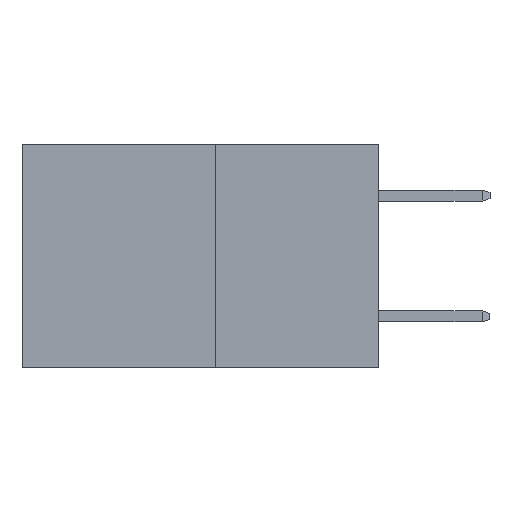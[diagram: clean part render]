
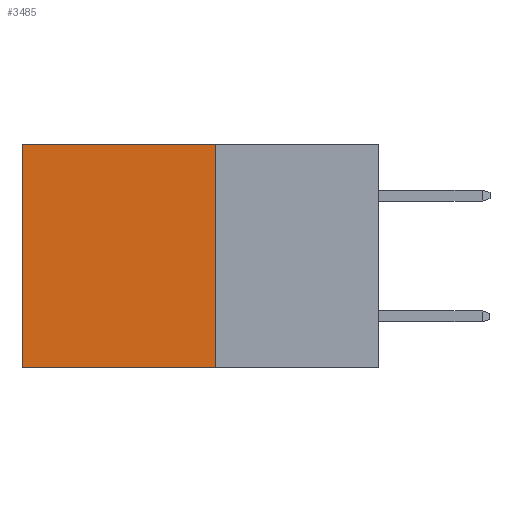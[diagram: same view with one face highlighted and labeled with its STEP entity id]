
A CAD part, left-side view. The second image highlights one B-rep face of the part: STEP entity #3485.
In plain terms, the highlighted planar face has unit normal (-1, 0, 0).
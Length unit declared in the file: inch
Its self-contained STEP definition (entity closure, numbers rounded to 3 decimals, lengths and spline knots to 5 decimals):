
#40 = DIRECTION ( 'NONE',  ( 1., 0., 0. ) ) ;
#182 = VECTOR ( 'NONE', #1301, 39.37008 ) ;
#316 = ORIENTED_EDGE ( 'NONE', *, *, #8505, .F. ) ;
#333 = VERTEX_POINT ( 'NONE', #3322 ) ;
#630 = EDGE_CURVE ( 'NONE', #333, #5329, #3388, .T. ) ;
#726 = DIRECTION ( 'NONE',  ( 0., 0., -1. ) ) ;
#749 = CARTESIAN_POINT ( 'NONE',  ( 0.277, 0.59, -0.37 ) ) ;
#883 = PLANE ( 'NONE',  #1421 ) ;
#895 = ORIENTED_EDGE ( 'NONE', *, *, #630, .F. ) ;
#913 = VECTOR ( 'NONE', #3841, 39.37008 ) ;
#981 = FACE_OUTER_BOUND ( 'NONE', #1476, .T. ) ;
#1301 = DIRECTION ( 'NONE',  ( 0., 0., -1. ) ) ;
#1337 = CARTESIAN_POINT ( 'NONE',  ( 0.277, 0.27, -0.37 ) ) ;
#1421 = AXIS2_PLACEMENT_3D ( 'NONE', #5021, #40, #4043 ) ;
#1476 = EDGE_LOOP ( 'NONE', ( #1556, #895, #316, #3253 ) ) ;
#1556 = ORIENTED_EDGE ( 'NONE', *, *, #6549, .T. ) ;
#2044 = LINE ( 'NONE', #1337, #182 ) ;
#2513 = VECTOR ( 'NONE', #4285, 39.37008 ) ;
#2818 = VECTOR ( 'NONE', #726, 39.37008 ) ;
#3253 = ORIENTED_EDGE ( 'NONE', *, *, #3258, .T. ) ;
#3258 = EDGE_CURVE ( 'NONE', #5971, #7368, #4491, .T. ) ;
#3322 = CARTESIAN_POINT ( 'NONE',  ( 0.277, 0.27, -0.37 ) ) ;
#3388 = LINE ( 'NONE', #4667, #913 ) ;
#3485 = ADVANCED_FACE ( 'NONE', ( #981 ), #883, .F. ) ;
#3841 = DIRECTION ( 'NONE',  ( 0., 1., 0. ) ) ;
#4043 = DIRECTION ( 'NONE',  ( 0., 0., -1. ) ) ;
#4285 = DIRECTION ( 'NONE',  ( 0., 1., 0. ) ) ;
#4491 = LINE ( 'NONE', #7439, #2513 ) ;
#4667 = CARTESIAN_POINT ( 'NONE',  ( 0.277, 0.27, -0.37 ) ) ;
#5021 = CARTESIAN_POINT ( 'NONE',  ( 0.277, 0.27, -0.37 ) ) ;
#5329 = VERTEX_POINT ( 'NONE', #8574 ) ;
#5820 = CARTESIAN_POINT ( 'NONE',  ( 0.277, 0.27, 0. ) ) ;
#5971 = VERTEX_POINT ( 'NONE', #5820 ) ;
#6151 = LINE ( 'NONE', #749, #2818 ) ;
#6549 = EDGE_CURVE ( 'NONE', #7368, #5329, #6151, .T. ) ;
#7368 = VERTEX_POINT ( 'NONE', #7788 ) ;
#7439 = CARTESIAN_POINT ( 'NONE',  ( 0.277, 0.27, 0. ) ) ;
#7788 = CARTESIAN_POINT ( 'NONE',  ( 0.277, 0.59, 0. ) ) ;
#8505 = EDGE_CURVE ( 'NONE', #5971, #333, #2044, .T. ) ;
#8574 = CARTESIAN_POINT ( 'NONE',  ( 0.277, 0.59, -0.37 ) ) ;
